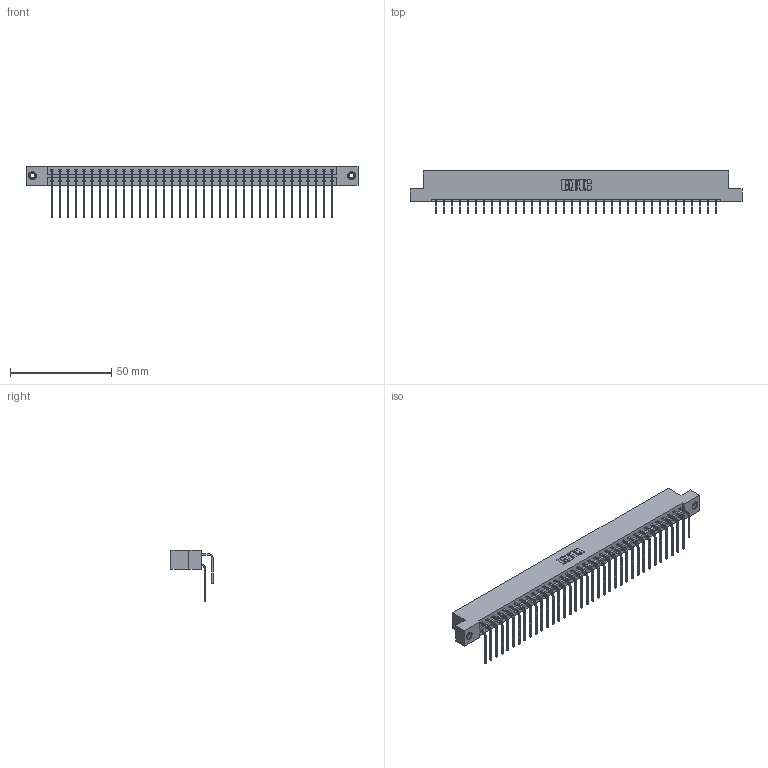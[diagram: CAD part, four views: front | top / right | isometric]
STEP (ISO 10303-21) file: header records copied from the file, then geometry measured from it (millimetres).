
FILE_DESCRIPTION (( 'STEP AP203' ), '1' );
FILE_NAME ('333-072-559-208.STEP', '2018-08-04T21:17:38', ( '' ), ( '' ), 'SwSTEP 2.0', 'SolidWorks 2016', '' );
FILE_SCHEMA (( 'CONFIG_CONTROL_DESIGN' ));
Length unit declared in the file: inch
Products named in the file (5): 345-292-001_558 559 Tail - 1; 345-292-001_559 Tail - 2; 345-250-001_345-250-003-102; 333-072-559-208; 333 Part_Flush - .156 Dia - TI
Assembly tree (75 placements, depth 2):
  333-072-559-208
    333 Part_Flush - .156 Dia - TI
    345-292-001_558 559 Tail - 1  x36
    345-292-001_559 Tail - 2  x36
    345-250-001_345-250-003-102  x2
Bounding box: 164.19 x 20.9 x 25.53 mm (x, y, z)
Volume: 17115.1 mm3; surface area: 22260.5 mm2
Topology: 75 solids, 75 shells, 4062 faces, 12039 edges, 7922 vertices
Faces by surface type: plane 2838, cylinder 1208, cone 12, torus 4
Entity records: 26906 total; most frequent: CARTESIAN_POINT 4500, ORIENTED_EDGE 4378, DIRECTION 3867, EDGE_CURVE 2189, VECTOR 2001, LINE 2001, VERTEX_POINT 1452, AXIS2_PLACEMENT_3D 933
